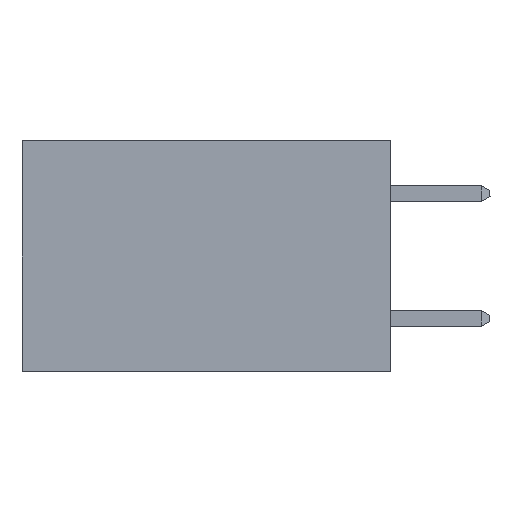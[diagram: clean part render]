
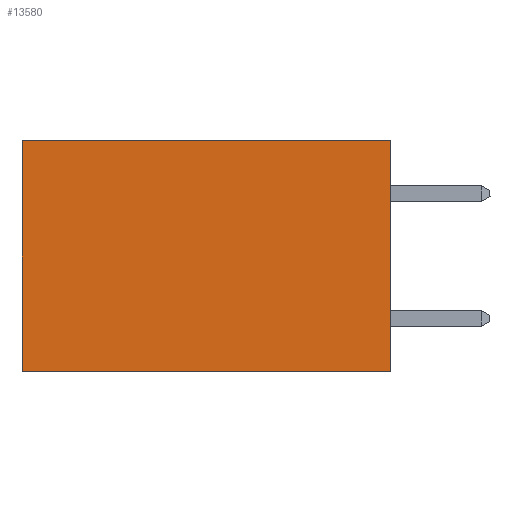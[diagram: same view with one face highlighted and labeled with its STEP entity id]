
A CAD part, left-side view. The second image highlights one B-rep face of the part: STEP entity #13580.
In plain terms, the highlighted planar face has unit normal (-1, 0, 0).
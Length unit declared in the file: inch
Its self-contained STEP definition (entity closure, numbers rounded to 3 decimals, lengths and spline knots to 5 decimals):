
#203 = CARTESIAN_POINT ( 'NONE',  ( 0.277, 0., -0.37 ) ) ;
#556 = CARTESIAN_POINT ( 'NONE',  ( 0.277, 0.59, 0. ) ) ;
#576 = ORIENTED_EDGE ( 'NONE', *, *, #12692, .T. ) ;
#655 = LINE ( 'NONE', #203, #1933 ) ;
#663 = EDGE_CURVE ( 'NONE', #24827, #18369, #10436, .T. ) ;
#1576 = CARTESIAN_POINT ( 'NONE',  ( 0.277, 0., 0. ) ) ;
#1933 = VECTOR ( 'NONE', #14431, 39.37008 ) ;
#2040 = EDGE_CURVE ( 'NONE', #24827, #11433, #25746, .T. ) ;
#2112 = DIRECTION ( 'NONE',  ( 0., 0., -1. ) ) ;
#4292 = AXIS2_PLACEMENT_3D ( 'NONE', #12263, #14288, #2112 ) ;
#4981 = VERTEX_POINT ( 'NONE', #18577 ) ;
#5158 = CARTESIAN_POINT ( 'NONE',  ( 0.277, 0., 0. ) ) ;
#5210 = FACE_OUTER_BOUND ( 'NONE', #5859, .T. ) ;
#5476 = ORIENTED_EDGE ( 'NONE', *, *, #2040, .T. ) ;
#5859 = EDGE_LOOP ( 'NONE', ( #576, #8352, #11795, #5476 ) ) ;
#5903 = LINE ( 'NONE', #19664, #11979 ) ;
#8352 = ORIENTED_EDGE ( 'NONE', *, *, #20435, .F. ) ;
#10436 = LINE ( 'NONE', #22532, #15204 ) ;
#11433 = VERTEX_POINT ( 'NONE', #556 ) ;
#11795 = ORIENTED_EDGE ( 'NONE', *, *, #663, .F. ) ;
#11979 = VECTOR ( 'NONE', #23685, 39.37008 ) ;
#12263 = CARTESIAN_POINT ( 'NONE',  ( 0.277, 0., -0.37 ) ) ;
#12692 = EDGE_CURVE ( 'NONE', #11433, #4981, #5903, .T. ) ;
#13580 = ADVANCED_FACE ( 'NONE', ( #5210 ), #24264, .F. ) ;
#14288 = DIRECTION ( 'NONE',  ( 1., 0., 0. ) ) ;
#14431 = DIRECTION ( 'NONE',  ( 0., 1., 0. ) ) ;
#15126 = VECTOR ( 'NONE', #21280, 39.37008 ) ;
#15204 = VECTOR ( 'NONE', #22893, 39.37008 ) ;
#18369 = VERTEX_POINT ( 'NONE', #23944 ) ;
#18577 = CARTESIAN_POINT ( 'NONE',  ( 0.277, 0.59, -0.37 ) ) ;
#19664 = CARTESIAN_POINT ( 'NONE',  ( 0.277, 0.59, -0.37 ) ) ;
#20435 = EDGE_CURVE ( 'NONE', #18369, #4981, #655, .T. ) ;
#21280 = DIRECTION ( 'NONE',  ( 0., 1., 0. ) ) ;
#22532 = CARTESIAN_POINT ( 'NONE',  ( 0.277, 0., -0.37 ) ) ;
#22893 = DIRECTION ( 'NONE',  ( 0., 0., -1. ) ) ;
#23685 = DIRECTION ( 'NONE',  ( 0., 0., -1. ) ) ;
#23944 = CARTESIAN_POINT ( 'NONE',  ( 0.277, 0., -0.37 ) ) ;
#24264 = PLANE ( 'NONE',  #4292 ) ;
#24827 = VERTEX_POINT ( 'NONE', #1576 ) ;
#25746 = LINE ( 'NONE', #5158, #15126 ) ;
